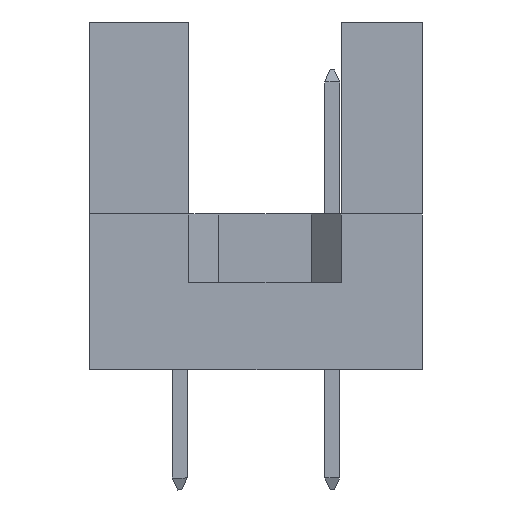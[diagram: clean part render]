
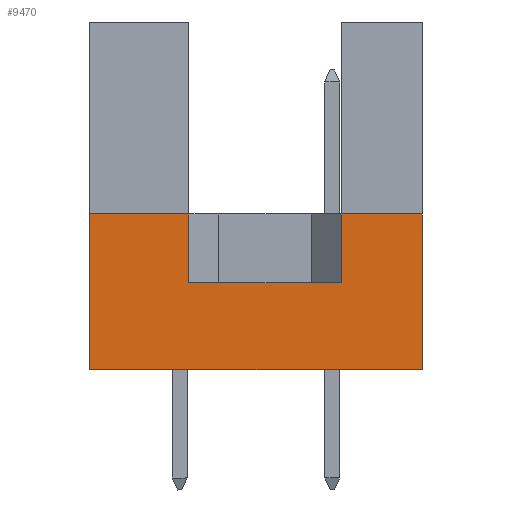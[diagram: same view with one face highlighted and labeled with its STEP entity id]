
A CAD part, left-side view. The second image highlights one B-rep face of the part: STEP entity #9470.
In plain terms, the highlighted planar face has unit normal (-1, 0, 0).
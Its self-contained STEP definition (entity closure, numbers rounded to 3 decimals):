
#183 = VECTOR ( 'NONE', #1986, 1000. ) ;
#363 = VERTEX_POINT ( 'NONE', #6810 ) ;
#600 = CARTESIAN_POINT ( 'NONE',  ( -47.5, 7.79, 2.9 ) ) ;
#629 = VECTOR ( 'NONE', #1879, 1000. ) ;
#766 = LINE ( 'NONE', #9525, #4512 ) ;
#974 = LINE ( 'NONE', #2127, #13120 ) ;
#1087 = LINE ( 'NONE', #12265, #9378 ) ;
#1101 = VERTEX_POINT ( 'NONE', #7689 ) ;
#1531 = VERTEX_POINT ( 'NONE', #14439 ) ;
#1879 = DIRECTION ( 'NONE',  ( 0., 0., 1. ) ) ;
#1896 = CARTESIAN_POINT ( 'NONE',  ( -47.5, 0., 0. ) ) ;
#1986 = DIRECTION ( 'NONE',  ( 0., 0., 1. ) ) ;
#2127 = CARTESIAN_POINT ( 'NONE',  ( -47.5, 11.1, 5.2 ) ) ;
#2362 = ORIENTED_EDGE ( 'NONE', *, *, #14584, .F. ) ;
#2883 = ORIENTED_EDGE ( 'NONE', *, *, #10555, .T. ) ;
#3524 = ORIENTED_EDGE ( 'NONE', *, *, #12804, .F. ) ;
#3630 = VERTEX_POINT ( 'NONE', #12387 ) ;
#4415 = DIRECTION ( 'NONE',  ( 0., 0., 1. ) ) ;
#4512 = VECTOR ( 'NONE', #4571, 1000. ) ;
#4525 = EDGE_CURVE ( 'NONE', #1101, #363, #766, .T. ) ;
#4543 = LINE ( 'NONE', #11898, #183 ) ;
#4571 = DIRECTION ( 'NONE',  ( 0., -1., 0. ) ) ;
#4836 = ORIENTED_EDGE ( 'NONE', *, *, #9216, .F. ) ;
#4999 = CARTESIAN_POINT ( 'NONE',  ( -47.5, 0., 5.2 ) ) ;
#5213 = VERTEX_POINT ( 'NONE', #1896 ) ;
#5679 = CARTESIAN_POINT ( 'NONE',  ( -47.5, 2.71, 2.9 ) ) ;
#5840 = CARTESIAN_POINT ( 'NONE',  ( -47.5, 2.71, 5.2 ) ) ;
#5977 = ORIENTED_EDGE ( 'NONE', *, *, #4525, .F. ) ;
#6084 = ORIENTED_EDGE ( 'NONE', *, *, #10982, .T. ) ;
#6802 = LINE ( 'NONE', #600, #9869 ) ;
#6810 = CARTESIAN_POINT ( 'NONE',  ( -47.5, 2.71, 2.9 ) ) ;
#6973 = DIRECTION ( 'NONE',  ( 0., -1., 0. ) ) ;
#6993 = ORIENTED_EDGE ( 'NONE', *, *, #10091, .T. ) ;
#7689 = CARTESIAN_POINT ( 'NONE',  ( -47.5, 7.79, 2.9 ) ) ;
#7825 = DIRECTION ( 'NONE',  ( 0., 0., -1. ) ) ;
#7867 = VERTEX_POINT ( 'NONE', #5840 ) ;
#8073 = VERTEX_POINT ( 'NONE', #11145 ) ;
#8208 = LINE ( 'NONE', #13275, #11986 ) ;
#8576 = DIRECTION ( 'NONE',  ( 0., -1., 0. ) ) ;
#8686 = DIRECTION ( 'NONE',  ( 0., -1., 0. ) ) ;
#8785 = AXIS2_PLACEMENT_3D ( 'NONE', #14134, #9224, #7825 ) ;
#8807 = CARTESIAN_POINT ( 'NONE',  ( -47.5, 0., 0. ) ) ;
#9064 = PLANE ( 'NONE',  #8785 ) ;
#9216 = EDGE_CURVE ( 'NONE', #363, #7867, #13395, .T. ) ;
#9224 = DIRECTION ( 'NONE',  ( 1., 0., 0. ) ) ;
#9338 = VECTOR ( 'NONE', #15201, 1000. ) ;
#9378 = VECTOR ( 'NONE', #8686, 1000. ) ;
#9470 = ADVANCED_FACE ( 'NONE', ( #10400 ), #9064, .F. ) ;
#9525 = CARTESIAN_POINT ( 'NONE',  ( -47.5, 7.79, 2.9 ) ) ;
#9869 = VECTOR ( 'NONE', #4415, 1000. ) ;
#10091 = EDGE_CURVE ( 'NONE', #1101, #1531, #6802, .T. ) ;
#10400 = FACE_OUTER_BOUND ( 'NONE', #15546, .T. ) ;
#10555 = EDGE_CURVE ( 'NONE', #5213, #14703, #16361, .T. ) ;
#10982 = EDGE_CURVE ( 'NONE', #3630, #5213, #8208, .T. ) ;
#11145 = CARTESIAN_POINT ( 'NONE',  ( -47.5, 11.1, 5.2 ) ) ;
#11898 = CARTESIAN_POINT ( 'NONE',  ( -47.5, 11.1, 0. ) ) ;
#11986 = VECTOR ( 'NONE', #6973, 1000. ) ;
#12265 = CARTESIAN_POINT ( 'NONE',  ( -47.5, 11.1, 5.2 ) ) ;
#12387 = CARTESIAN_POINT ( 'NONE',  ( -47.5, 11.1, 0. ) ) ;
#12804 = EDGE_CURVE ( 'NONE', #8073, #1531, #1087, .T. ) ;
#13120 = VECTOR ( 'NONE', #8576, 1000. ) ;
#13275 = CARTESIAN_POINT ( 'NONE',  ( -47.5, 11.1, 0. ) ) ;
#13395 = LINE ( 'NONE', #5679, #629 ) ;
#14134 = CARTESIAN_POINT ( 'NONE',  ( -47.5, 11.1, 0. ) ) ;
#14439 = CARTESIAN_POINT ( 'NONE',  ( -47.5, 7.79, 5.2 ) ) ;
#14584 = EDGE_CURVE ( 'NONE', #7867, #14703, #974, .T. ) ;
#14703 = VERTEX_POINT ( 'NONE', #4999 ) ;
#15034 = EDGE_CURVE ( 'NONE', #3630, #8073, #4543, .T. ) ;
#15201 = DIRECTION ( 'NONE',  ( 0., 0., 1. ) ) ;
#15546 = EDGE_LOOP ( 'NONE', ( #5977, #6993, #3524, #15809, #6084, #2883, #2362, #4836 ) ) ;
#15809 = ORIENTED_EDGE ( 'NONE', *, *, #15034, .F. ) ;
#16361 = LINE ( 'NONE', #8807, #9338 ) ;
